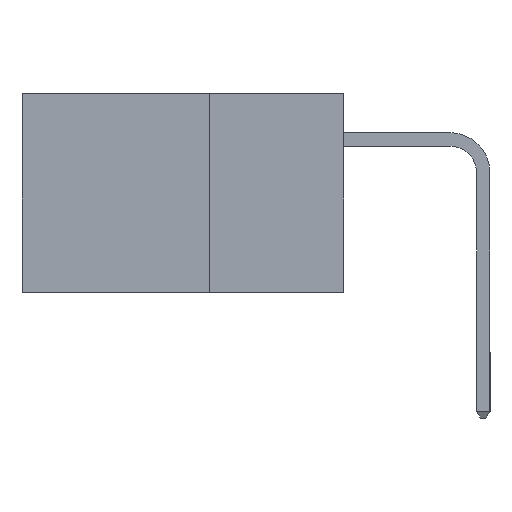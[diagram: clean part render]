
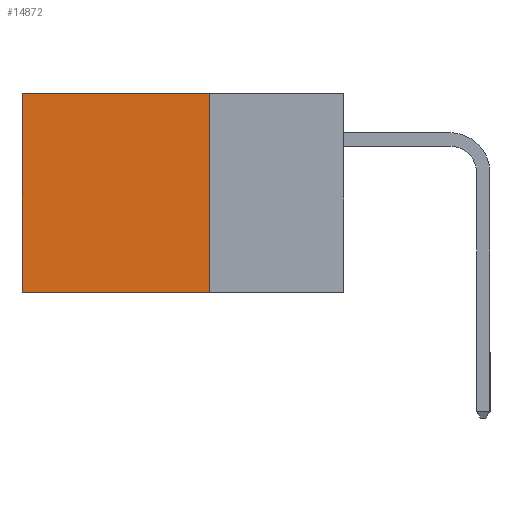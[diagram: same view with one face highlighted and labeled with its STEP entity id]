
A CAD part, left-side view. The second image highlights one B-rep face of the part: STEP entity #14872.
In plain terms, the highlighted planar face has unit normal (-1, 0, 0).
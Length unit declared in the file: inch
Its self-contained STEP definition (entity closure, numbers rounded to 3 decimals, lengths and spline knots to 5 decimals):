
#143 = DIRECTION ( 'NONE',  ( 0., 0., -1. ) ) ;
#193 = VECTOR ( 'NONE', #143, 39.37008 ) ;
#433 = PLANE ( 'NONE',  #9696 ) ;
#835 = LINE ( 'NONE', #19462, #17925 ) ;
#878 = LINE ( 'NONE', #8722, #193 ) ;
#1468 = CARTESIAN_POINT ( 'NONE',  ( 0.298, 0.6, 0. ) ) ;
#2577 = DIRECTION ( 'NONE',  ( 1., 0., 0. ) ) ;
#5385 = DIRECTION ( 'NONE',  ( 0., 1., 0. ) ) ;
#6239 = LINE ( 'NONE', #18746, #22594 ) ;
#6674 = DIRECTION ( 'NONE',  ( 0., 1., 0. ) ) ;
#7069 = EDGE_CURVE ( 'NONE', #22251, #11059, #12914, .T. ) ;
#7834 = FACE_OUTER_BOUND ( 'NONE', #20668, .T. ) ;
#7927 = VECTOR ( 'NONE', #5385, 39.37008 ) ;
#8722 = CARTESIAN_POINT ( 'NONE',  ( 0.298, 0.25, 0. ) ) ;
#9696 = AXIS2_PLACEMENT_3D ( 'NONE', #15433, #2577, #17569 ) ;
#11059 = VERTEX_POINT ( 'NONE', #16848 ) ;
#11105 = CARTESIAN_POINT ( 'NONE',  ( 0.298, 0.25, -0.37 ) ) ;
#12441 = ORIENTED_EDGE ( 'NONE', *, *, #22872, .T. ) ;
#12852 = EDGE_CURVE ( 'NONE', #16285, #22251, #878, .T. ) ;
#12914 = LINE ( 'NONE', #16061, #7927 ) ;
#14552 = DIRECTION ( 'NONE',  ( 0., 0., -1. ) ) ;
#14872 = ADVANCED_FACE ( 'NONE', ( #7834 ), #433, .F. ) ;
#15433 = CARTESIAN_POINT ( 'NONE',  ( 0.298, 0.25, 0. ) ) ;
#16061 = CARTESIAN_POINT ( 'NONE',  ( 0.298, 0.25, -0.37 ) ) ;
#16285 = VERTEX_POINT ( 'NONE', #25682 ) ;
#16848 = CARTESIAN_POINT ( 'NONE',  ( 0.298, 0.6, -0.37 ) ) ;
#17569 = DIRECTION ( 'NONE',  ( 0., 0., -1. ) ) ;
#17925 = VECTOR ( 'NONE', #6674, 39.37008 ) ;
#18224 = ORIENTED_EDGE ( 'NONE', *, *, #12852, .F. ) ;
#18746 = CARTESIAN_POINT ( 'NONE',  ( 0.298, 0.6, 0. ) ) ;
#19462 = CARTESIAN_POINT ( 'NONE',  ( 0.298, 0.25, 0. ) ) ;
#20108 = ORIENTED_EDGE ( 'NONE', *, *, #21989, .T. ) ;
#20668 = EDGE_LOOP ( 'NONE', ( #20108, #25726, #18224, #12441 ) ) ;
#21989 = EDGE_CURVE ( 'NONE', #26383, #11059, #6239, .T. ) ;
#22251 = VERTEX_POINT ( 'NONE', #11105 ) ;
#22594 = VECTOR ( 'NONE', #14552, 39.37008 ) ;
#22872 = EDGE_CURVE ( 'NONE', #16285, #26383, #835, .T. ) ;
#25682 = CARTESIAN_POINT ( 'NONE',  ( 0.298, 0.25, 0. ) ) ;
#25726 = ORIENTED_EDGE ( 'NONE', *, *, #7069, .F. ) ;
#26383 = VERTEX_POINT ( 'NONE', #1468 ) ;
